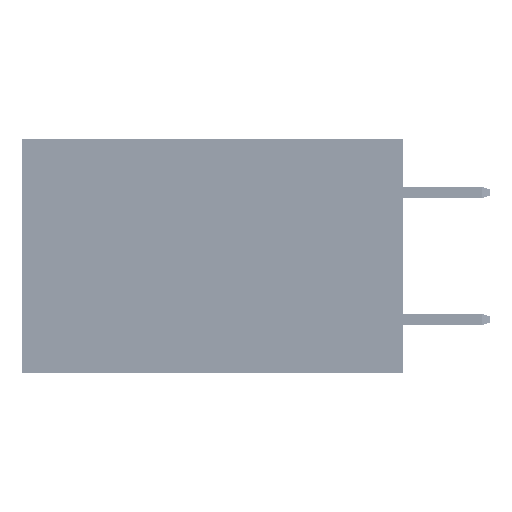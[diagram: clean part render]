
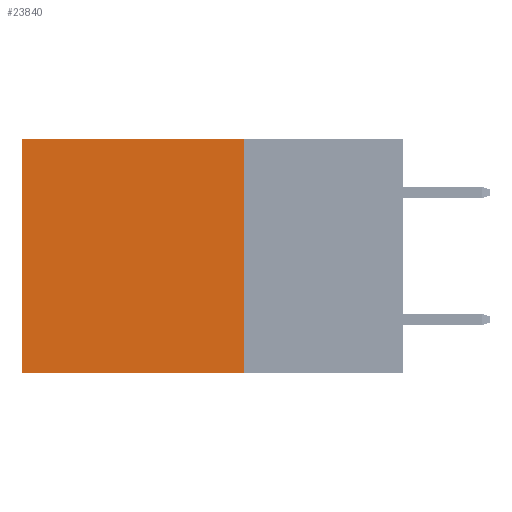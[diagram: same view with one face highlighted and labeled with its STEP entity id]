
A CAD part, left-side view. The second image highlights one B-rep face of the part: STEP entity #23840.
In plain terms, the highlighted planar face has unit normal (-1, 0, 0).
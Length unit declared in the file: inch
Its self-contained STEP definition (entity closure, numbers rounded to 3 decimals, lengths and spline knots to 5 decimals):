
#1069 = VECTOR ( 'NONE', #12678, 39.37008 ) ;
#1073 = VERTEX_POINT ( 'NONE', #43275 ) ;
#2509 = LINE ( 'NONE', #46317, #36224 ) ;
#2682 = EDGE_CURVE ( 'NONE', #23455, #1073, #13197, .T. ) ;
#4013 = CARTESIAN_POINT ( 'NONE',  ( 0.2875, 0.25, 0. ) ) ;
#7325 = EDGE_LOOP ( 'NONE', ( #21803, #13736, #9885, #13501 ) ) ;
#8702 = CARTESIAN_POINT ( 'NONE',  ( 0.2875, 0.25, 0. ) ) ;
#9885 = ORIENTED_EDGE ( 'NONE', *, *, #44202, .F. ) ;
#11942 = FACE_OUTER_BOUND ( 'NONE', #7325, .T. ) ;
#12652 = CARTESIAN_POINT ( 'NONE',  ( 0.2875, 0.25, 0. ) ) ;
#12678 = DIRECTION ( 'NONE',  ( 0., 1., 0. ) ) ;
#13197 = LINE ( 'NONE', #8702, #1069 ) ;
#13501 = ORIENTED_EDGE ( 'NONE', *, *, #2682, .T. ) ;
#13736 = ORIENTED_EDGE ( 'NONE', *, *, #51970, .F. ) ;
#16251 = VECTOR ( 'NONE', #28845, 39.37008 ) ;
#17240 = AXIS2_PLACEMENT_3D ( 'NONE', #4013, #20184, #36373 ) ;
#18682 = DIRECTION ( 'NONE',  ( 0., 0., -1. ) ) ;
#18767 = CARTESIAN_POINT ( 'NONE',  ( 0.2875, 0.6, -0.37 ) ) ;
#20184 = DIRECTION ( 'NONE',  ( 1., 0., 0. ) ) ;
#21803 = ORIENTED_EDGE ( 'NONE', *, *, #36955, .T. ) ;
#21811 = CARTESIAN_POINT ( 'NONE',  ( 0.2875, 0.25, -0.37 ) ) ;
#23455 = VERTEX_POINT ( 'NONE', #49705 ) ;
#23840 = ADVANCED_FACE ( 'NONE', ( #11942 ), #28142, .F. ) ;
#28142 = PLANE ( 'NONE',  #17240 ) ;
#28845 = DIRECTION ( 'NONE',  ( 0., 0., -1. ) ) ;
#33082 = LINE ( 'NONE', #12652, #16251 ) ;
#35429 = VERTEX_POINT ( 'NONE', #38321 ) ;
#36224 = VECTOR ( 'NONE', #18682, 39.37008 ) ;
#36373 = DIRECTION ( 'NONE',  ( 0., 0., -1. ) ) ;
#36955 = EDGE_CURVE ( 'NONE', #1073, #39893, #2509, .T. ) ;
#38025 = DIRECTION ( 'NONE',  ( 0., 1., 0. ) ) ;
#38321 = CARTESIAN_POINT ( 'NONE',  ( 0.2875, 0.25, -0.37 ) ) ;
#39893 = VERTEX_POINT ( 'NONE', #18767 ) ;
#40448 = VECTOR ( 'NONE', #38025, 39.37008 ) ;
#43275 = CARTESIAN_POINT ( 'NONE',  ( 0.2875, 0.6, 0. ) ) ;
#44202 = EDGE_CURVE ( 'NONE', #23455, #35429, #33082, .T. ) ;
#46317 = CARTESIAN_POINT ( 'NONE',  ( 0.2875, 0.6, 0. ) ) ;
#49705 = CARTESIAN_POINT ( 'NONE',  ( 0.2875, 0.25, 0. ) ) ;
#51970 = EDGE_CURVE ( 'NONE', #35429, #39893, #52050, .T. ) ;
#52050 = LINE ( 'NONE', #21811, #40448 ) ;
